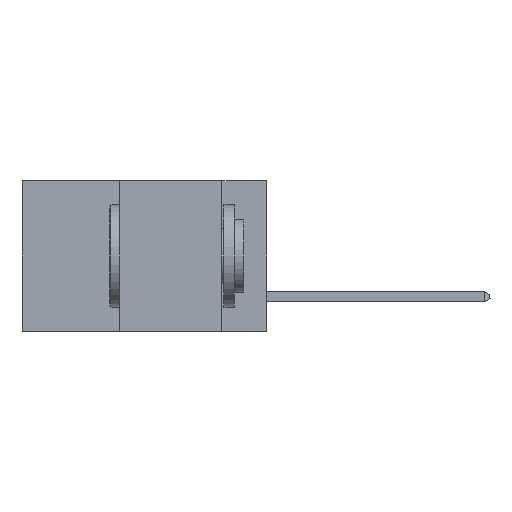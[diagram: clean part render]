
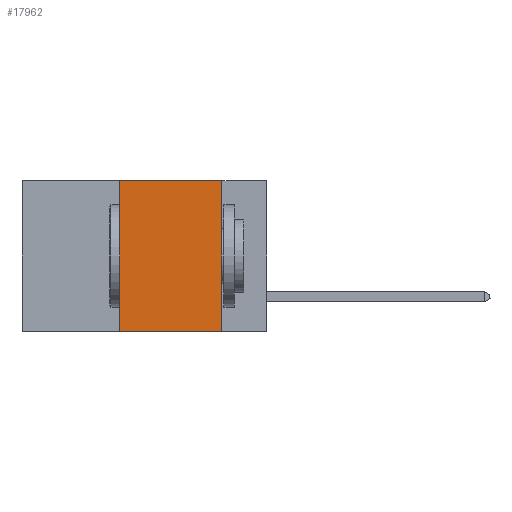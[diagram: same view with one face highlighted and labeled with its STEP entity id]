
A CAD part, left-side view. The second image highlights one B-rep face of the part: STEP entity #17962.
In plain terms, the highlighted planar face has unit normal (-1, 0, 0).
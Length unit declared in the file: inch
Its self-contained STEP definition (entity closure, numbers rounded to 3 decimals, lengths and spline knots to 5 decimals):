
#161 = DIRECTION ( 'NONE',  ( 0., -1., 0. ) ) ;
#361 = LINE ( 'NONE', #8487, #18852 ) ;
#780 = VECTOR ( 'NONE', #18768, 39.37008 ) ;
#1409 = VERTEX_POINT ( 'NONE', #14562 ) ;
#2500 = VERTEX_POINT ( 'NONE', #15548 ) ;
#2683 = FACE_OUTER_BOUND ( 'NONE', #3677, .T. ) ;
#2972 = EDGE_CURVE ( 'NONE', #1409, #2500, #3863, .T. ) ;
#3677 = EDGE_LOOP ( 'NONE', ( #11301, #11662, #12026, #19991 ) ) ;
#3863 = LINE ( 'NONE', #20029, #12551 ) ;
#4593 = VERTEX_POINT ( 'NONE', #5139 ) ;
#5139 = CARTESIAN_POINT ( 'NONE',  ( 0., 0.11, 0. ) ) ;
#5769 = CARTESIAN_POINT ( 'NONE',  ( 0., 0.36, 0. ) ) ;
#6602 = DIRECTION ( 'NONE',  ( 1., 0., 0. ) ) ;
#7564 = DIRECTION ( 'NONE',  ( 0., 0., 1. ) ) ;
#8487 = CARTESIAN_POINT ( 'NONE',  ( 0., 0.6, 0. ) ) ;
#9353 = LINE ( 'NONE', #5769, #10763 ) ;
#9484 = LINE ( 'NONE', #22169, #780 ) ;
#9564 = AXIS2_PLACEMENT_3D ( 'NONE', #13431, #6602, #17099 ) ;
#10662 = CARTESIAN_POINT ( 'NONE',  ( 0., 0.36, 0. ) ) ;
#10763 = VECTOR ( 'NONE', #7564, 39.37008 ) ;
#11301 = ORIENTED_EDGE ( 'NONE', *, *, #22779, .F. ) ;
#11662 = ORIENTED_EDGE ( 'NONE', *, *, #14839, .F. ) ;
#11744 = VERTEX_POINT ( 'NONE', #10662 ) ;
#12026 = ORIENTED_EDGE ( 'NONE', *, *, #19710, .F. ) ;
#12535 = PLANE ( 'NONE',  #9564 ) ;
#12551 = VECTOR ( 'NONE', #161, 39.37008 ) ;
#13431 = CARTESIAN_POINT ( 'NONE',  ( 0., 0.6, 0. ) ) ;
#14562 = CARTESIAN_POINT ( 'NONE',  ( 0., 0.36, -0.37 ) ) ;
#14839 = EDGE_CURVE ( 'NONE', #11744, #4593, #361, .T. ) ;
#15548 = CARTESIAN_POINT ( 'NONE',  ( 0., 0.11, -0.37 ) ) ;
#17099 = DIRECTION ( 'NONE',  ( 0., 0., -1. ) ) ;
#17962 = ADVANCED_FACE ( 'NONE', ( #2683 ), #12535, .F. ) ;
#18768 = DIRECTION ( 'NONE',  ( 0., 0., -1. ) ) ;
#18852 = VECTOR ( 'NONE', #21302, 39.37008 ) ;
#19710 = EDGE_CURVE ( 'NONE', #1409, #11744, #9353, .T. ) ;
#19991 = ORIENTED_EDGE ( 'NONE', *, *, #2972, .T. ) ;
#20029 = CARTESIAN_POINT ( 'NONE',  ( 0., 0.6, -0.37 ) ) ;
#21302 = DIRECTION ( 'NONE',  ( 0., -1., 0. ) ) ;
#22169 = CARTESIAN_POINT ( 'NONE',  ( 0., 0.11, 0. ) ) ;
#22779 = EDGE_CURVE ( 'NONE', #4593, #2500, #9484, .T. ) ;
